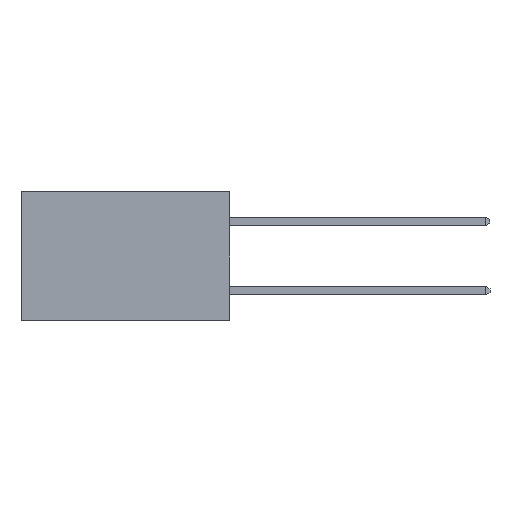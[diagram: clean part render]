
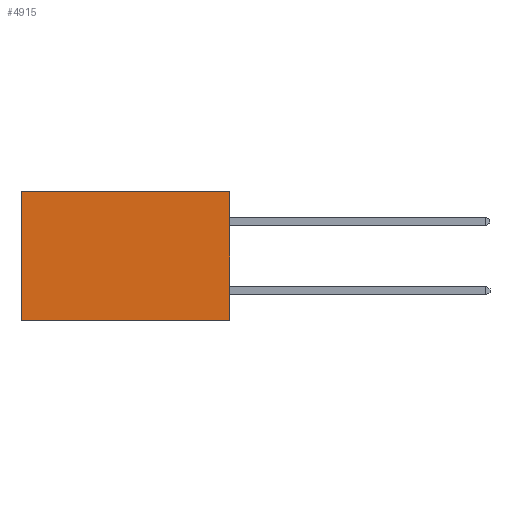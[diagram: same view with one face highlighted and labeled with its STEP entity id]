
A CAD part, left-side view. The second image highlights one B-rep face of the part: STEP entity #4915.
In plain terms, the highlighted planar face has unit normal (-1, 0, 0).
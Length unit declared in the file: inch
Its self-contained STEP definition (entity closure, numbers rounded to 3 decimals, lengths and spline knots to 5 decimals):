
#67 = CARTESIAN_POINT ( 'NONE',  ( 0.2615, 0.6, -0.37 ) ) ;
#107 = LINE ( 'NONE', #4235, #12034 ) ;
#483 = EDGE_CURVE ( 'NONE', #1449, #14346, #107, .T. ) ;
#495 = EDGE_LOOP ( 'NONE', ( #831, #4947, #7808, #13233 ) ) ;
#831 = ORIENTED_EDGE ( 'NONE', *, *, #5478, .T. ) ;
#1302 = DIRECTION ( 'NONE',  ( 0., 0., -1. ) ) ;
#1324 = VECTOR ( 'NONE', #1561, 39.37008 ) ;
#1449 = VERTEX_POINT ( 'NONE', #13128 ) ;
#1495 = CARTESIAN_POINT ( 'NONE',  ( 0.2615, 0., -0.37 ) ) ;
#1561 = DIRECTION ( 'NONE',  ( 0., 1., 0. ) ) ;
#1672 = CARTESIAN_POINT ( 'NONE',  ( 0.2615, 0., -0.37 ) ) ;
#2658 = LINE ( 'NONE', #1672, #1324 ) ;
#3020 = EDGE_CURVE ( 'NONE', #1449, #11017, #5283, .T. ) ;
#3774 = AXIS2_PLACEMENT_3D ( 'NONE', #7442, #7426, #7410 ) ;
#4012 = EDGE_CURVE ( 'NONE', #14346, #7347, #2658, .T. ) ;
#4235 = CARTESIAN_POINT ( 'NONE',  ( 0.2615, 0., -0.37 ) ) ;
#4915 = ADVANCED_FACE ( 'NONE', ( #10383 ), #7542, .F. ) ;
#4947 = ORIENTED_EDGE ( 'NONE', *, *, #4012, .F. ) ;
#4981 = VECTOR ( 'NONE', #5898, 39.37008 ) ;
#5283 = LINE ( 'NONE', #13292, #12879 ) ;
#5478 = EDGE_CURVE ( 'NONE', #11017, #7347, #7834, .T. ) ;
#5898 = DIRECTION ( 'NONE',  ( 0., 0., -1. ) ) ;
#6705 = CARTESIAN_POINT ( 'NONE',  ( 0.2615, 0.6, -0.37 ) ) ;
#7347 = VERTEX_POINT ( 'NONE', #67 ) ;
#7410 = DIRECTION ( 'NONE',  ( 0., 0., -1. ) ) ;
#7426 = DIRECTION ( 'NONE',  ( 1., 0., 0. ) ) ;
#7442 = CARTESIAN_POINT ( 'NONE',  ( 0.2615, 0., -0.37 ) ) ;
#7542 = PLANE ( 'NONE',  #3774 ) ;
#7730 = CARTESIAN_POINT ( 'NONE',  ( 0.2615, 0.6, 0. ) ) ;
#7808 = ORIENTED_EDGE ( 'NONE', *, *, #483, .F. ) ;
#7834 = LINE ( 'NONE', #6705, #4981 ) ;
#10383 = FACE_OUTER_BOUND ( 'NONE', #495, .T. ) ;
#11017 = VERTEX_POINT ( 'NONE', #7730 ) ;
#12034 = VECTOR ( 'NONE', #1302, 39.37008 ) ;
#12879 = VECTOR ( 'NONE', #13181, 39.37008 ) ;
#13128 = CARTESIAN_POINT ( 'NONE',  ( 0.2615, 0., 0. ) ) ;
#13181 = DIRECTION ( 'NONE',  ( 0., 1., 0. ) ) ;
#13233 = ORIENTED_EDGE ( 'NONE', *, *, #3020, .T. ) ;
#13292 = CARTESIAN_POINT ( 'NONE',  ( 0.2615, 0., 0. ) ) ;
#14346 = VERTEX_POINT ( 'NONE', #1495 ) ;
